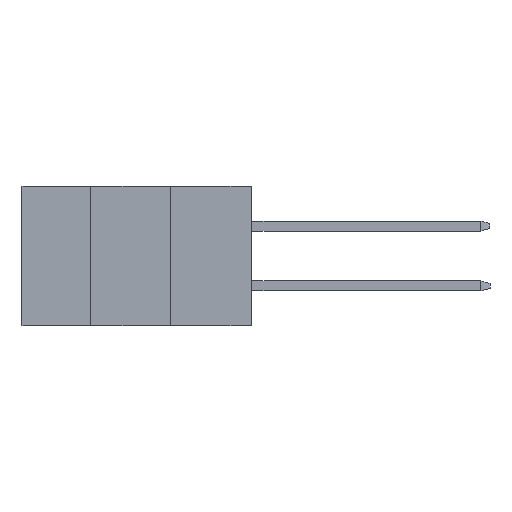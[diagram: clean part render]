
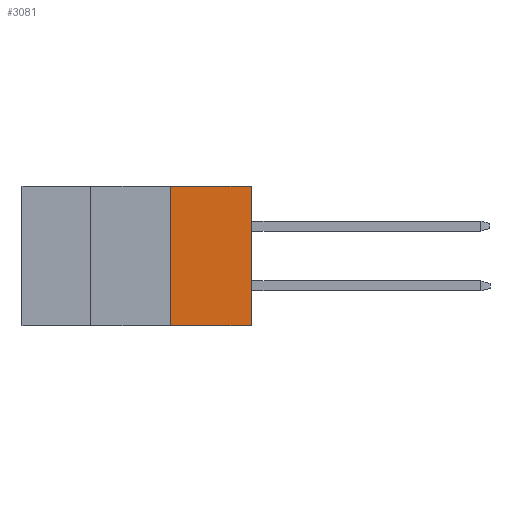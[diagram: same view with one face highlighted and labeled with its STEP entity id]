
A CAD part, left-side view. The second image highlights one B-rep face of the part: STEP entity #3081.
In plain terms, the highlighted planar face has unit normal (-1, 0, 0).
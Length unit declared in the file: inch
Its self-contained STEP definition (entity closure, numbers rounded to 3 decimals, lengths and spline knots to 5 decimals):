
#562 = LINE ( 'NONE', #6410, #9341 ) ;
#1073 = DIRECTION ( 'NONE',  ( 0., 0., 1. ) ) ;
#1286 = CARTESIAN_POINT ( 'NONE',  ( 0.4265, 0., -0.437 ) ) ;
#2064 = VECTOR ( 'NONE', #4047, 39.37008 ) ;
#2342 = CARTESIAN_POINT ( 'NONE',  ( 0.4265, 0., 0. ) ) ;
#3037 = EDGE_CURVE ( 'NONE', #18461, #5157, #8218, .T. ) ;
#3081 = ADVANCED_FACE ( 'NONE', ( #3646 ), #12911, .F. ) ;
#3646 = FACE_OUTER_BOUND ( 'NONE', #9364, .T. ) ;
#4047 = DIRECTION ( 'NONE',  ( 0., -1., 0. ) ) ;
#4499 = EDGE_CURVE ( 'NONE', #11546, #12495, #8323, .T. ) ;
#5157 = VERTEX_POINT ( 'NONE', #2342 ) ;
#5247 = ORIENTED_EDGE ( 'NONE', *, *, #15822, .F. ) ;
#5407 = CARTESIAN_POINT ( 'NONE',  ( 0.4265, 0.254, -0.437 ) ) ;
#6115 = ORIENTED_EDGE ( 'NONE', *, *, #4499, .T. ) ;
#6410 = CARTESIAN_POINT ( 'NONE',  ( 0.4265, 0.254, -0.437 ) ) ;
#7009 = CARTESIAN_POINT ( 'NONE',  ( 0.4265, 0.254, 0. ) ) ;
#8079 = EDGE_CURVE ( 'NONE', #12495, #5157, #8777, .T. ) ;
#8177 = DIRECTION ( 'NONE',  ( 0., 0., 1. ) ) ;
#8218 = LINE ( 'NONE', #7009, #2064 ) ;
#8323 = LINE ( 'NONE', #15520, #17245 ) ;
#8777 = LINE ( 'NONE', #14793, #17411 ) ;
#9005 = AXIS2_PLACEMENT_3D ( 'NONE', #5407, #19027, #14105 ) ;
#9341 = VECTOR ( 'NONE', #8177, 39.37008 ) ;
#9364 = EDGE_LOOP ( 'NONE', ( #12945, #16908, #5247, #6115 ) ) ;
#10829 = CARTESIAN_POINT ( 'NONE',  ( 0.4265, 0.254, -0.437 ) ) ;
#11546 = VERTEX_POINT ( 'NONE', #10829 ) ;
#12495 = VERTEX_POINT ( 'NONE', #1286 ) ;
#12661 = DIRECTION ( 'NONE',  ( 0., -1., 0. ) ) ;
#12911 = PLANE ( 'NONE',  #9005 ) ;
#12945 = ORIENTED_EDGE ( 'NONE', *, *, #8079, .T. ) ;
#14105 = DIRECTION ( 'NONE',  ( 0., 0., -1. ) ) ;
#14793 = CARTESIAN_POINT ( 'NONE',  ( 0.4265, 0., -0.437 ) ) ;
#15520 = CARTESIAN_POINT ( 'NONE',  ( 0.4265, 0.254, -0.437 ) ) ;
#15822 = EDGE_CURVE ( 'NONE', #11546, #18461, #562, .T. ) ;
#16021 = CARTESIAN_POINT ( 'NONE',  ( 0.4265, 0.254, 0. ) ) ;
#16908 = ORIENTED_EDGE ( 'NONE', *, *, #3037, .F. ) ;
#17245 = VECTOR ( 'NONE', #12661, 39.37008 ) ;
#17411 = VECTOR ( 'NONE', #1073, 39.37008 ) ;
#18461 = VERTEX_POINT ( 'NONE', #16021 ) ;
#19027 = DIRECTION ( 'NONE',  ( 1., 0., 0. ) ) ;
